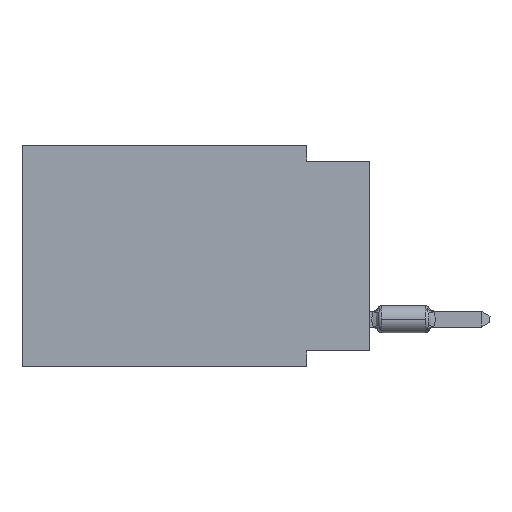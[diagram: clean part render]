
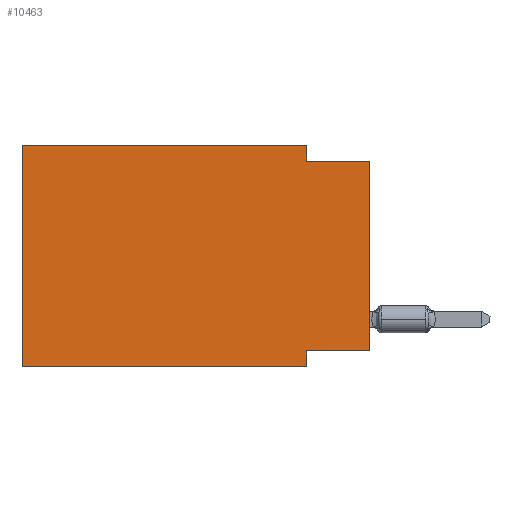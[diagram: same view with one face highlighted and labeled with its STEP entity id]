
A CAD part, left-side view. The second image highlights one B-rep face of the part: STEP entity #10463.
In plain terms, the highlighted planar face has unit normal (-1, 0, 0).
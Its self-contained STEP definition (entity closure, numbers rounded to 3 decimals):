
#248 = DIRECTION ( 'NONE',  ( 0., -1., 0. ) ) ;
#421 = VECTOR ( 'NONE', #15315, 1000. ) ;
#447 = VERTEX_POINT ( 'NONE', #16211 ) ;
#1436 = ORIENTED_EDGE ( 'NONE', *, *, #11114, .F. ) ;
#1494 = VERTEX_POINT ( 'NONE', #17486 ) ;
#1529 = DIRECTION ( 'NONE',  ( 0., 0., -1. ) ) ;
#1917 = LINE ( 'NONE', #7686, #3235 ) ;
#1979 = ORIENTED_EDGE ( 'NONE', *, *, #13393, .F. ) ;
#2155 = VERTEX_POINT ( 'NONE', #8615 ) ;
#2260 = FACE_OUTER_BOUND ( 'NONE', #14112, .T. ) ;
#2645 = DIRECTION ( 'NONE',  ( 0., 1., 0. ) ) ;
#2646 = CARTESIAN_POINT ( 'NONE',  ( 0., 2.54, 0. ) ) ;
#2869 = VECTOR ( 'NONE', #2645, 1000. ) ;
#3159 = LINE ( 'NONE', #16585, #16584 ) ;
#3235 = VECTOR ( 'NONE', #14457, 1000. ) ;
#4057 = VERTEX_POINT ( 'NONE', #9837 ) ;
#4140 = DIRECTION ( 'NONE',  ( 0., 0., -1. ) ) ;
#4323 = LINE ( 'NONE', #15302, #13063 ) ;
#4337 = CARTESIAN_POINT ( 'NONE',  ( 0., 13.97, -8.89 ) ) ;
#4439 = EDGE_CURVE ( 'NONE', #447, #12676, #7536, .T. ) ;
#4993 = CARTESIAN_POINT ( 'NONE',  ( 0., 13.97, 0. ) ) ;
#5153 = VERTEX_POINT ( 'NONE', #12911 ) ;
#5315 = DIRECTION ( 'NONE',  ( 1., 0., 0. ) ) ;
#5443 = LINE ( 'NONE', #16427, #5923 ) ;
#5836 = VERTEX_POINT ( 'NONE', #14862 ) ;
#5923 = VECTOR ( 'NONE', #10175, 1000. ) ;
#5984 = EDGE_CURVE ( 'NONE', #1494, #12676, #9809, .T. ) ;
#6555 = EDGE_CURVE ( 'NONE', #12587, #5153, #5443, .T. ) ;
#7093 = EDGE_CURVE ( 'NONE', #1494, #4057, #3159, .T. ) ;
#7426 = ORIENTED_EDGE ( 'NONE', *, *, #5984, .T. ) ;
#7536 = LINE ( 'NONE', #8977, #12513 ) ;
#7686 = CARTESIAN_POINT ( 'NONE',  ( 0., 13.97, 0. ) ) ;
#8183 = ORIENTED_EDGE ( 'NONE', *, *, #6555, .F. ) ;
#8615 = CARTESIAN_POINT ( 'NONE',  ( 0., 0., -8.255 ) ) ;
#8692 = EDGE_CURVE ( 'NONE', #5153, #5836, #4323, .T. ) ;
#8864 = AXIS2_PLACEMENT_3D ( 'NONE', #4993, #5315, #4140 ) ;
#8977 = CARTESIAN_POINT ( 'NONE',  ( 0., 2.54, -8.89 ) ) ;
#9220 = ORIENTED_EDGE ( 'NONE', *, *, #7093, .F. ) ;
#9244 = CARTESIAN_POINT ( 'NONE',  ( 0., 0., 0. ) ) ;
#9486 = LINE ( 'NONE', #16177, #2869 ) ;
#9563 = ORIENTED_EDGE ( 'NONE', *, *, #4439, .F. ) ;
#9809 = LINE ( 'NONE', #4337, #421 ) ;
#9837 = CARTESIAN_POINT ( 'NONE',  ( 0., 13.97, 0. ) ) ;
#10175 = DIRECTION ( 'NONE',  ( 0., 0., -1. ) ) ;
#10463 = ADVANCED_FACE ( 'NONE', ( #2260 ), #17829, .F. ) ;
#10841 = EDGE_CURVE ( 'NONE', #2155, #5836, #14830, .T. ) ;
#11026 = ORIENTED_EDGE ( 'NONE', *, *, #8692, .F. ) ;
#11114 = EDGE_CURVE ( 'NONE', #4057, #12587, #1917, .T. ) ;
#11560 = VECTOR ( 'NONE', #17714, 1000. ) ;
#12513 = VECTOR ( 'NONE', #1529, 1000. ) ;
#12524 = DIRECTION ( 'NONE',  ( 0., 0., 1. ) ) ;
#12587 = VERTEX_POINT ( 'NONE', #2646 ) ;
#12676 = VERTEX_POINT ( 'NONE', #13901 ) ;
#12911 = CARTESIAN_POINT ( 'NONE',  ( 0., 2.54, -0.635 ) ) ;
#13063 = VECTOR ( 'NONE', #248, 1000. ) ;
#13393 = EDGE_CURVE ( 'NONE', #2155, #447, #9486, .T. ) ;
#13901 = CARTESIAN_POINT ( 'NONE',  ( 0., 2.54, -8.89 ) ) ;
#14112 = EDGE_LOOP ( 'NONE', ( #15677, #11026, #8183, #1436, #9220, #7426, #9563, #1979 ) ) ;
#14457 = DIRECTION ( 'NONE',  ( 0., -1., 0. ) ) ;
#14830 = LINE ( 'NONE', #9244, #11560 ) ;
#14862 = CARTESIAN_POINT ( 'NONE',  ( 0., 0., -0.635 ) ) ;
#15302 = CARTESIAN_POINT ( 'NONE',  ( 0., 0., -0.635 ) ) ;
#15315 = DIRECTION ( 'NONE',  ( 0., -1., 0. ) ) ;
#15677 = ORIENTED_EDGE ( 'NONE', *, *, #10841, .T. ) ;
#16177 = CARTESIAN_POINT ( 'NONE',  ( 0., 0., -8.255 ) ) ;
#16211 = CARTESIAN_POINT ( 'NONE',  ( 0., 2.54, -8.255 ) ) ;
#16427 = CARTESIAN_POINT ( 'NONE',  ( 0., 2.54, 0. ) ) ;
#16584 = VECTOR ( 'NONE', #12524, 1000. ) ;
#16585 = CARTESIAN_POINT ( 'NONE',  ( 0., 13.97, 0. ) ) ;
#17486 = CARTESIAN_POINT ( 'NONE',  ( 0., 13.97, -8.89 ) ) ;
#17714 = DIRECTION ( 'NONE',  ( 0., 0., 1. ) ) ;
#17829 = PLANE ( 'NONE',  #8864 ) ;
